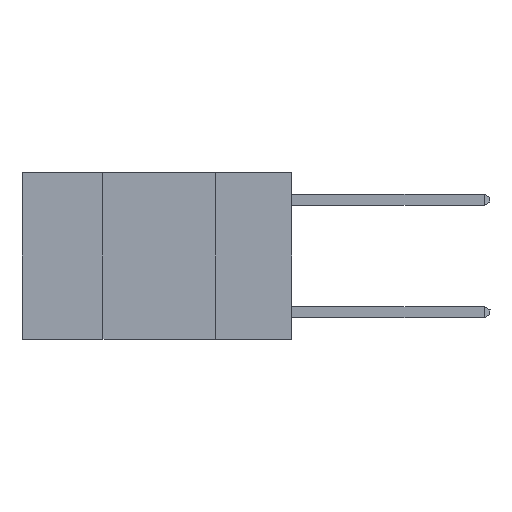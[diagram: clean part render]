
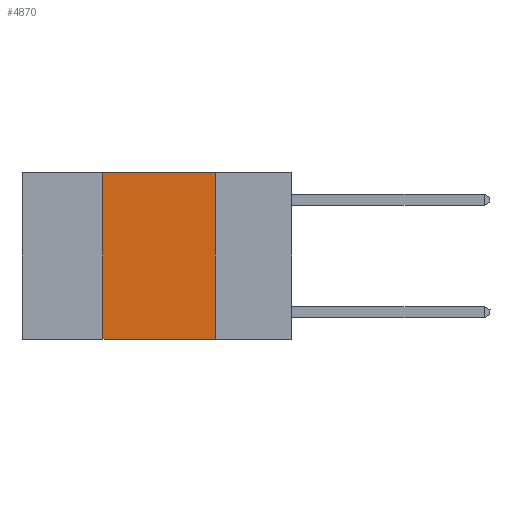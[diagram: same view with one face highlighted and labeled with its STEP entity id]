
A CAD part, left-side view. The second image highlights one B-rep face of the part: STEP entity #4870.
In plain terms, the highlighted planar face has unit normal (-1, 0, 0).
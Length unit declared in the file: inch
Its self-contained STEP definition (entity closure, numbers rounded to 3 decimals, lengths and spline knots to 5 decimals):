
#190 = CARTESIAN_POINT ( 'NONE',  ( 0., 0.17, 0. ) ) ;
#432 = VERTEX_POINT ( 'NONE', #190 ) ;
#711 = LINE ( 'NONE', #6153, #5198 ) ;
#951 = CARTESIAN_POINT ( 'NONE',  ( 0., 0.42, -0.37 ) ) ;
#984 = DIRECTION ( 'NONE',  ( 0., -1., 0. ) ) ;
#1102 = EDGE_CURVE ( 'NONE', #2072, #3029, #1418, .T. ) ;
#1418 = LINE ( 'NONE', #4471, #10794 ) ;
#1755 = CARTESIAN_POINT ( 'NONE',  ( 0., 0.17, 0. ) ) ;
#1775 = CARTESIAN_POINT ( 'NONE',  ( 0., 0.42, 0. ) ) ;
#1845 = DIRECTION ( 'NONE',  ( 0., 0., -1. ) ) ;
#2072 = VERTEX_POINT ( 'NONE', #951 ) ;
#2263 = EDGE_CURVE ( 'NONE', #432, #3029, #7788, .T. ) ;
#2776 = DIRECTION ( 'NONE',  ( 0., 0., -1. ) ) ;
#3029 = VERTEX_POINT ( 'NONE', #7027 ) ;
#3454 = EDGE_CURVE ( 'NONE', #2072, #8553, #5921, .T. ) ;
#3607 = CARTESIAN_POINT ( 'NONE',  ( 0., 0.6, 0. ) ) ;
#4471 = CARTESIAN_POINT ( 'NONE',  ( 0., 0.6, -0.37 ) ) ;
#4507 = EDGE_LOOP ( 'NONE', ( #10621, #6028, #6741, #5864 ) ) ;
#4830 = AXIS2_PLACEMENT_3D ( 'NONE', #3607, #7142, #1845 ) ;
#4870 = ADVANCED_FACE ( 'NONE', ( #7339 ), #10623, .F. ) ;
#5198 = VECTOR ( 'NONE', #5268, 39.37008 ) ;
#5268 = DIRECTION ( 'NONE',  ( 0., -1., 0. ) ) ;
#5385 = CARTESIAN_POINT ( 'NONE',  ( 0., 0.42, 0. ) ) ;
#5864 = ORIENTED_EDGE ( 'NONE', *, *, #1102, .T. ) ;
#5921 = LINE ( 'NONE', #5385, #8309 ) ;
#6028 = ORIENTED_EDGE ( 'NONE', *, *, #7877, .F. ) ;
#6153 = CARTESIAN_POINT ( 'NONE',  ( 0., 0.6, 0. ) ) ;
#6741 = ORIENTED_EDGE ( 'NONE', *, *, #3454, .F. ) ;
#7027 = CARTESIAN_POINT ( 'NONE',  ( 0., 0.17, -0.37 ) ) ;
#7142 = DIRECTION ( 'NONE',  ( 1., 0., 0. ) ) ;
#7339 = FACE_OUTER_BOUND ( 'NONE', #4507, .T. ) ;
#7519 = VECTOR ( 'NONE', #2776, 39.37008 ) ;
#7788 = LINE ( 'NONE', #1755, #7519 ) ;
#7877 = EDGE_CURVE ( 'NONE', #8553, #432, #711, .T. ) ;
#8309 = VECTOR ( 'NONE', #10378, 39.37008 ) ;
#8553 = VERTEX_POINT ( 'NONE', #1775 ) ;
#10378 = DIRECTION ( 'NONE',  ( 0., 0., 1. ) ) ;
#10621 = ORIENTED_EDGE ( 'NONE', *, *, #2263, .F. ) ;
#10623 = PLANE ( 'NONE',  #4830 ) ;
#10794 = VECTOR ( 'NONE', #984, 39.37008 ) ;
